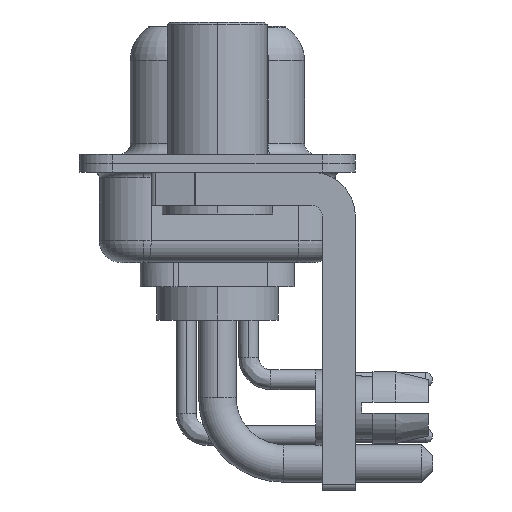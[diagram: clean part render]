
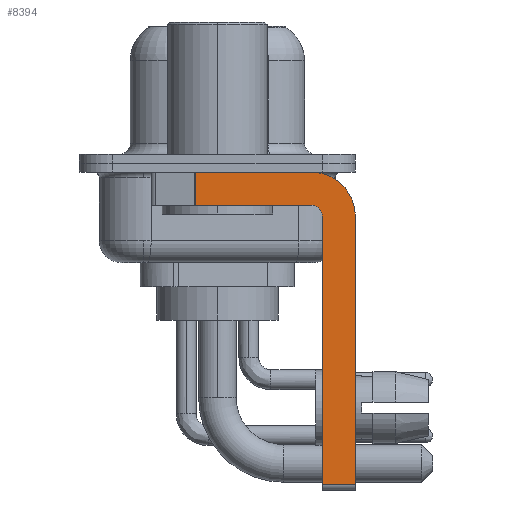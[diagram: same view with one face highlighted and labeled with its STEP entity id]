
A CAD part, left-side view. The second image highlights one B-rep face of the part: STEP entity #8394.
In plain terms, the highlighted planar face has unit normal (-1, 0, 0).
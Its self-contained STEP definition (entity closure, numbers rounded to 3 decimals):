
#148 = CARTESIAN_POINT ( 'NONE',  ( -2.9, -4.25, -1.9 ) ) ;
#536 = DIRECTION ( 'NONE',  ( 0., 0., -1. ) ) ;
#2585 = PLANE ( 'NONE',  #3892 ) ;
#2875 = CARTESIAN_POINT ( 'NONE',  ( -2.9, -4.25, -14.55 ) ) ;
#2927 = CARTESIAN_POINT ( 'NONE',  ( -2.9, -4.25, -2.4 ) ) ;
#2928 = CARTESIAN_POINT ( 'NONE',  ( -2.9, -6.25, -14.55 ) ) ;
#3227 = VECTOR ( 'NONE', #12883, 1000. ) ;
#3892 = AXIS2_PLACEMENT_3D ( 'NONE', #15374, #13683, #17169 ) ;
#5500 = VERTEX_POINT ( 'NONE', #2928 ) ;
#5681 = CARTESIAN_POINT ( 'NONE',  ( -2.9, 0.978, -1.9 ) ) ;
#5966 = CARTESIAN_POINT ( 'NONE',  ( -2.9, -4.75, -2.4 ) ) ;
#6179 = DIRECTION ( 'NONE',  ( 0., 0., -1. ) ) ;
#6512 = ORIENTED_EDGE ( 'NONE', *, *, #20917, .F. ) ;
#7055 = VERTEX_POINT ( 'NONE', #5681 ) ;
#7479 = EDGE_CURVE ( 'NONE', #13218, #5500, #15234, .T. ) ;
#7497 = FACE_OUTER_BOUND ( 'NONE', #12031, .T. ) ;
#7500 = VECTOR ( 'NONE', #20988, 1000. ) ;
#7676 = DIRECTION ( 'NONE',  ( 1., 0., 0. ) ) ;
#7884 = CARTESIAN_POINT ( 'NONE',  ( -2.9, -4.75, -14.8 ) ) ;
#7981 = VERTEX_POINT ( 'NONE', #13526 ) ;
#8066 = ORIENTED_EDGE ( 'NONE', *, *, #18386, .T. ) ;
#8394 = ADVANCED_FACE ( 'NONE', ( #7497 ), #2585, .F. ) ;
#8454 = CARTESIAN_POINT ( 'NONE',  ( -2.9, -4.25, -1.9 ) ) ;
#8636 = ORIENTED_EDGE ( 'NONE', *, *, #8830, .F. ) ;
#8648 = CARTESIAN_POINT ( 'NONE',  ( -2.9, 0.978, -1.9 ) ) ;
#8830 = EDGE_CURVE ( 'NONE', #7981, #19652, #17868, .T. ) ;
#9205 = ORIENTED_EDGE ( 'NONE', *, *, #18477, .F. ) ;
#9439 = DIRECTION ( 'NONE',  ( -1., 0., 0. ) ) ;
#9497 = DIRECTION ( 'NONE',  ( 0., -1., 0. ) ) ;
#9534 = CARTESIAN_POINT ( 'NONE',  ( -2.9, -4.25, -0.4 ) ) ;
#10179 = CIRCLE ( 'NONE', #12215, 0.5 ) ;
#10351 = VECTOR ( 'NONE', #15455, 1000. ) ;
#10428 = ORIENTED_EDGE ( 'NONE', *, *, #15065, .F. ) ;
#11305 = VECTOR ( 'NONE', #9497, 1000. ) ;
#11506 = VERTEX_POINT ( 'NONE', #17346 ) ;
#11724 = LINE ( 'NONE', #8648, #14366 ) ;
#12031 = EDGE_LOOP ( 'NONE', ( #14126, #15073, #6512, #10428, #8636, #8066, #18646, #9205 ) ) ;
#12215 = AXIS2_PLACEMENT_3D ( 'NONE', #2927, #9439, #20273 ) ;
#12883 = DIRECTION ( 'NONE',  ( 0., 0., 1. ) ) ;
#13218 = VERTEX_POINT ( 'NONE', #19667 ) ;
#13526 = CARTESIAN_POINT ( 'NONE',  ( -2.9, -4.75, -14.55 ) ) ;
#13683 = DIRECTION ( 'NONE',  ( 1., 0., 0. ) ) ;
#13756 = CARTESIAN_POINT ( 'NONE',  ( -2.9, -6.25, -2.4 ) ) ;
#14126 = ORIENTED_EDGE ( 'NONE', *, *, #16665, .F. ) ;
#14267 = CARTESIAN_POINT ( 'NONE',  ( -2.9, -4.25, -2.4 ) ) ;
#14366 = VECTOR ( 'NONE', #536, 1000. ) ;
#14509 = CARTESIAN_POINT ( 'NONE',  ( -2.9, 3., -0.4 ) ) ;
#15065 = EDGE_CURVE ( 'NONE', #19652, #18169, #10179, .T. ) ;
#15073 = ORIENTED_EDGE ( 'NONE', *, *, #20084, .T. ) ;
#15234 = LINE ( 'NONE', #13756, #10351 ) ;
#15374 = CARTESIAN_POINT ( 'NONE',  ( -2.9, -4.25, -2.4 ) ) ;
#15455 = DIRECTION ( 'NONE',  ( 0., 0., -1. ) ) ;
#15727 = AXIS2_PLACEMENT_3D ( 'NONE', #14267, #7676, #6179 ) ;
#15737 = VECTOR ( 'NONE', #21000, 1000. ) ;
#16665 = EDGE_CURVE ( 'NONE', #11506, #20893, #19271, .T. ) ;
#17169 = DIRECTION ( 'NONE',  ( 0., 0., -1. ) ) ;
#17346 = CARTESIAN_POINT ( 'NONE',  ( -2.9, 0.978, -0.4 ) ) ;
#17584 = LINE ( 'NONE', #148, #15737 ) ;
#17868 = LINE ( 'NONE', #7884, #3227 ) ;
#18169 = VERTEX_POINT ( 'NONE', #8454 ) ;
#18386 = EDGE_CURVE ( 'NONE', #7981, #5500, #20863, .T. ) ;
#18477 = EDGE_CURVE ( 'NONE', #20893, #13218, #20147, .T. ) ;
#18646 = ORIENTED_EDGE ( 'NONE', *, *, #7479, .F. ) ;
#19271 = LINE ( 'NONE', #14509, #7500 ) ;
#19652 = VERTEX_POINT ( 'NONE', #5966 ) ;
#19667 = CARTESIAN_POINT ( 'NONE',  ( -2.9, -6.25, -2.4 ) ) ;
#20084 = EDGE_CURVE ( 'NONE', #11506, #7055, #11724, .T. ) ;
#20147 = CIRCLE ( 'NONE', #15727, 2. ) ;
#20273 = DIRECTION ( 'NONE',  ( 0., 0., 1. ) ) ;
#20863 = LINE ( 'NONE', #2875, #11305 ) ;
#20893 = VERTEX_POINT ( 'NONE', #9534 ) ;
#20917 = EDGE_CURVE ( 'NONE', #18169, #7055, #17584, .T. ) ;
#20988 = DIRECTION ( 'NONE',  ( 0., -1., 0. ) ) ;
#21000 = DIRECTION ( 'NONE',  ( 0., 1., 0. ) ) ;
